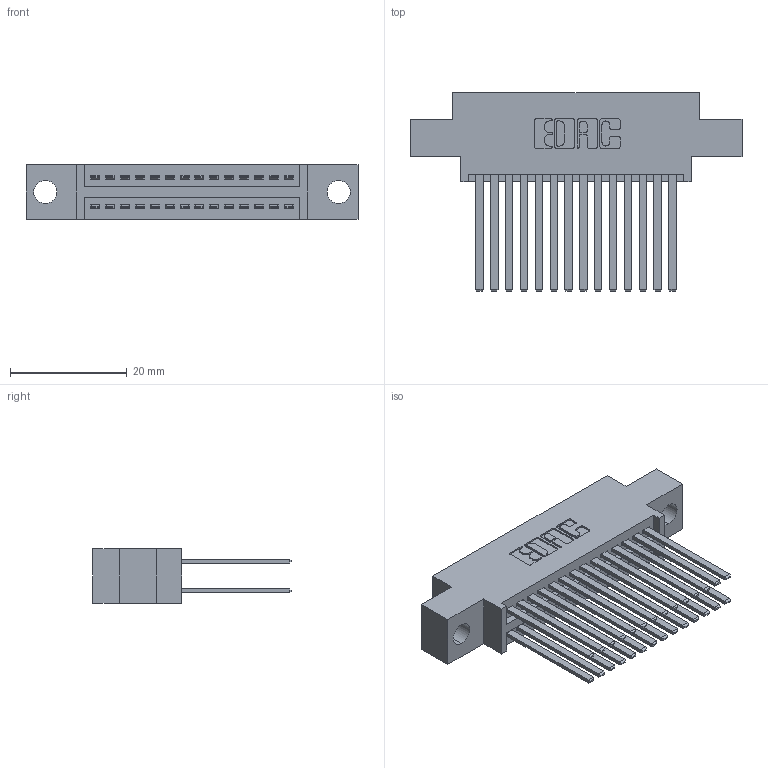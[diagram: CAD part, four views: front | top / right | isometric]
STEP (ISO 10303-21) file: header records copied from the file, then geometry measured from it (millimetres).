
FILE_DESCRIPTION (( 'STEP AP203' ), '1' );
FILE_NAME ('395-028-544-804.STEP', '2021-06-16T19:52:38', ( '' ), ( '' ), 'SwSTEP 2.0', 'SolidWorks 2020', '' );
FILE_SCHEMA (( 'CONFIG_CONTROL_DESIGN' ));
Length unit declared in the file: inch
Products named in the file (3): 345-292-001_345-293-144; 345 Part_0.170 Offset - 0.156 Dia-TI; 395-028-544-804
Assembly tree (29 placements, depth 2):
  395-028-544-804
    345 Part_0.170 Offset - 0.156 Dia-TI
    345-292-001_345-293-144  x28
Bounding box: 56.77 x 33.96 x 9.4 mm (x, y, z)
Volume: 5427.9 mm3; surface area: 8626.5 mm2
Topology: 29 solids, 29 shells, 1376 faces, 4057 edges, 2666 vertices
Faces by surface type: plane 910, cylinder 466
Entity records: 15121 total; most frequent: CARTESIAN_POINT 2566, ORIENTED_EDGE 2498, DIRECTION 2293, EDGE_CURVE 1249, LINE 1065, VECTOR 1065, VERTEX_POINT 830, AXIS2_PLACEMENT_3D 614
